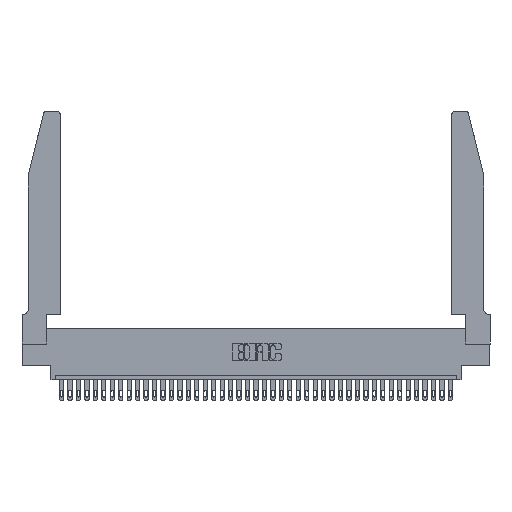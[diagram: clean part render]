
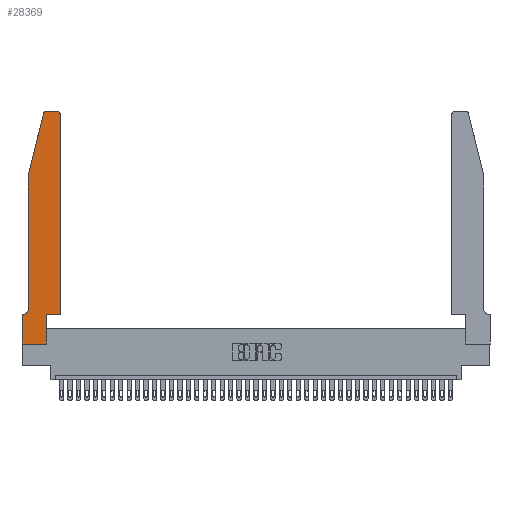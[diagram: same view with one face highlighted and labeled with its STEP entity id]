
A CAD part, top view. The second image highlights one B-rep face of the part: STEP entity #28369.
In plain terms, the highlighted planar face has unit normal (0, 0, 1).
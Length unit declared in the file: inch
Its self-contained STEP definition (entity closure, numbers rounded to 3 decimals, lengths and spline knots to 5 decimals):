
#581 = DIRECTION ( 'NONE',  ( 0., 0., 1. ) ) ;
#1126 = ORIENTED_EDGE ( 'NONE', *, *, #22174, .T. ) ;
#1524 = ORIENTED_EDGE ( 'NONE', *, *, #20832, .T. ) ;
#1776 = CARTESIAN_POINT ( 'NONE',  ( 0.0755, 2., 0.37 ) ) ;
#2032 = VERTEX_POINT ( 'NONE', #5130 ) ;
#2088 = CARTESIAN_POINT ( 'NONE',  ( 0.4505, 0.35, 0.37 ) ) ;
#2096 = CARTESIAN_POINT ( 'NONE',  ( 0.4205, 2.75, 0.37 ) ) ;
#2989 = EDGE_CURVE ( 'NONE', #11575, #21661, #34814, .T. ) ;
#3261 = CARTESIAN_POINT ( 'NONE',  ( 0., 0., 0.37 ) ) ;
#4809 = CARTESIAN_POINT ( 'NONE',  ( 0., 0., 0.37 ) ) ;
#5130 = CARTESIAN_POINT ( 'NONE',  ( 0.25487, 2.72718, 0.37 ) ) ;
#5205 = ORIENTED_EDGE ( 'NONE', *, *, #6544, .T. ) ;
#5489 = VECTOR ( 'NONE', #34188, 39.37008 ) ;
#5509 = DIRECTION ( 'NONE',  ( 0., 0., 1. ) ) ;
#5736 = EDGE_CURVE ( 'NONE', #28441, #7665, #14526, .T. ) ;
#6529 = LINE ( 'NONE', #38360, #15579 ) ;
#6544 = EDGE_CURVE ( 'NONE', #32827, #2032, #7242, .T. ) ;
#6547 = ORIENTED_EDGE ( 'NONE', *, *, #39200, .T. ) ;
#6992 = VERTEX_POINT ( 'NONE', #17213 ) ;
#7242 = CIRCLE ( 'NONE', #26897, 0.03 ) ;
#7665 = VERTEX_POINT ( 'NONE', #8176 ) ;
#7895 = AXIS2_PLACEMENT_3D ( 'NONE', #32499, #20428, #26489 ) ;
#8176 = CARTESIAN_POINT ( 'NONE',  ( 0.2865, 0., 0.37 ) ) ;
#8455 = ORIENTED_EDGE ( 'NONE', *, *, #27224, .T. ) ;
#8778 = LINE ( 'NONE', #24167, #14963 ) ;
#8881 = ORIENTED_EDGE ( 'NONE', *, *, #11420, .T. ) ;
#9319 = DIRECTION ( 'NONE',  ( 1., 0., 0. ) ) ;
#9985 = PLANE ( 'NONE',  #35301 ) ;
#10122 = CARTESIAN_POINT ( 'NONE',  ( 0., 0.35, 0.37 ) ) ;
#11025 = CARTESIAN_POINT ( 'NONE',  ( 0., 0., 0.37 ) ) ;
#11032 = ORIENTED_EDGE ( 'NONE', *, *, #2989, .T. ) ;
#11420 = EDGE_CURVE ( 'NONE', #21661, #14140, #14455, .T. ) ;
#11493 = CARTESIAN_POINT ( 'NONE',  ( 0.4205, 2.72, 0.37 ) ) ;
#11575 = VERTEX_POINT ( 'NONE', #30525 ) ;
#11626 = DIRECTION ( 'NONE',  ( 1., 0., 0. ) ) ;
#11891 = DIRECTION ( 'NONE',  ( 1., 0., 0. ) ) ;
#12230 = DIRECTION ( 'NONE',  ( 0., 1., 0. ) ) ;
#12401 = LINE ( 'NONE', #24390, #24803 ) ;
#12436 = DIRECTION ( 'NONE',  ( -0.239, -0.971, 0. ) ) ;
#12817 = CARTESIAN_POINT ( 'NONE',  ( 0.0755, 0.35, 0.37 ) ) ;
#13031 = DIRECTION ( 'NONE',  ( 1., 0., 0. ) ) ;
#13671 = EDGE_LOOP ( 'NONE', ( #31301, #5205, #18286, #1524, #35792, #8455, #6547, #36989, #1126, #28188, #11032, #8881 ) ) ;
#14140 = VERTEX_POINT ( 'NONE', #2096 ) ;
#14239 = VERTEX_POINT ( 'NONE', #30895 ) ;
#14455 = CIRCLE ( 'NONE', #35148, 0.03 ) ;
#14526 = LINE ( 'NONE', #3261, #29839 ) ;
#14963 = VECTOR ( 'NONE', #11891, 39.37008 ) ;
#15190 = VERTEX_POINT ( 'NONE', #31787 ) ;
#15579 = VECTOR ( 'NONE', #26239, 39.37008 ) ;
#17213 = CARTESIAN_POINT ( 'NONE',  ( 0.0055, 0.35, 0.37 ) ) ;
#18286 = ORIENTED_EDGE ( 'NONE', *, *, #27577, .T. ) ;
#18552 = VECTOR ( 'NONE', #26552, 39.37008 ) ;
#20428 = DIRECTION ( 'NONE',  ( 0., 0., -1. ) ) ;
#20656 = VECTOR ( 'NONE', #38276, 39.37008 ) ;
#20832 = EDGE_CURVE ( 'NONE', #37397, #14239, #26401, .T. ) ;
#21661 = VERTEX_POINT ( 'NONE', #24568 ) ;
#21700 = VERTEX_POINT ( 'NONE', #25064 ) ;
#22174 = EDGE_CURVE ( 'NONE', #7665, #21700, #12401, .T. ) ;
#23571 = VECTOR ( 'NONE', #12436, 39.37008 ) ;
#24167 = CARTESIAN_POINT ( 'NONE',  ( 0.4505, 0.35, 0.37 ) ) ;
#24390 = CARTESIAN_POINT ( 'NONE',  ( 0.2865, 0.35, 0.37 ) ) ;
#24525 = DIRECTION ( 'NONE',  ( 0., 0., 1. ) ) ;
#24568 = CARTESIAN_POINT ( 'NONE',  ( 0.4505, 2.72, 0.37 ) ) ;
#24625 = EDGE_CURVE ( 'NONE', #14140, #32827, #6529, .T. ) ;
#24803 = VECTOR ( 'NONE', #12230, 39.37008 ) ;
#25064 = CARTESIAN_POINT ( 'NONE',  ( 0.2865, 0.35, 0.37 ) ) ;
#25879 = CARTESIAN_POINT ( 'NONE',  ( 0.0755, 2., 0.37 ) ) ;
#25923 = VECTOR ( 'NONE', #28874, 39.37008 ) ;
#26239 = DIRECTION ( 'NONE',  ( -1., 0., 0. ) ) ;
#26401 = LINE ( 'NONE', #1776, #25923 ) ;
#26489 = DIRECTION ( 'NONE',  ( -1., 0., 0. ) ) ;
#26552 = DIRECTION ( 'NONE',  ( 0., 1., 0. ) ) ;
#26897 = AXIS2_PLACEMENT_3D ( 'NONE', #27024, #24525, #9319 ) ;
#27024 = CARTESIAN_POINT ( 'NONE',  ( 0.284, 2.72, 0.37 ) ) ;
#27224 = EDGE_CURVE ( 'NONE', #6992, #15190, #35589, .T. ) ;
#27433 = LINE ( 'NONE', #27452, #23571 ) ;
#27452 = CARTESIAN_POINT ( 'NONE',  ( 0.0755, 2., 0.37 ) ) ;
#27577 = EDGE_CURVE ( 'NONE', #2032, #37397, #27433, .T. ) ;
#28188 = ORIENTED_EDGE ( 'NONE', *, *, #38912, .T. ) ;
#28248 = EDGE_CURVE ( 'NONE', #14239, #6992, #33121, .T. ) ;
#28369 = ADVANCED_FACE ( 'NONE', ( #28795 ), #9985, .T. ) ;
#28441 = VERTEX_POINT ( 'NONE', #11025 ) ;
#28795 = FACE_OUTER_BOUND ( 'NONE', #13671, .T. ) ;
#28874 = DIRECTION ( 'NONE',  ( 0., -1., 0. ) ) ;
#29839 = VECTOR ( 'NONE', #36509, 39.37008 ) ;
#30525 = CARTESIAN_POINT ( 'NONE',  ( 0.4505, 0.35, 0.37 ) ) ;
#30895 = CARTESIAN_POINT ( 'NONE',  ( 0.0755, 0.42, 0.37 ) ) ;
#31301 = ORIENTED_EDGE ( 'NONE', *, *, #24625, .T. ) ;
#31787 = CARTESIAN_POINT ( 'NONE',  ( 0., 0.35, 0.37 ) ) ;
#31893 = CARTESIAN_POINT ( 'NONE',  ( 0.284, 2.75, 0.37 ) ) ;
#32499 = CARTESIAN_POINT ( 'NONE',  ( 0.0055, 0.42, 0.37 ) ) ;
#32827 = VERTEX_POINT ( 'NONE', #31893 ) ;
#33121 = CIRCLE ( 'NONE', #7895, 0.07 ) ;
#34188 = DIRECTION ( 'NONE',  ( -1., 0., 0. ) ) ;
#34814 = LINE ( 'NONE', #2088, #18552 ) ;
#35148 = AXIS2_PLACEMENT_3D ( 'NONE', #11493, #5509, #11626 ) ;
#35301 = AXIS2_PLACEMENT_3D ( 'NONE', #10122, #581, #13031 ) ;
#35485 = LINE ( 'NONE', #4809, #20656 ) ;
#35589 = LINE ( 'NONE', #12817, #5489 ) ;
#35792 = ORIENTED_EDGE ( 'NONE', *, *, #28248, .T. ) ;
#36509 = DIRECTION ( 'NONE',  ( 1., 0., 0. ) ) ;
#36989 = ORIENTED_EDGE ( 'NONE', *, *, #5736, .T. ) ;
#37397 = VERTEX_POINT ( 'NONE', #25879 ) ;
#38276 = DIRECTION ( 'NONE',  ( 0., -1., 0. ) ) ;
#38360 = CARTESIAN_POINT ( 'NONE',  ( 0.2605, 2.75, 0.37 ) ) ;
#38912 = EDGE_CURVE ( 'NONE', #21700, #11575, #8778, .T. ) ;
#39200 = EDGE_CURVE ( 'NONE', #15190, #28441, #35485, .T. ) ;
